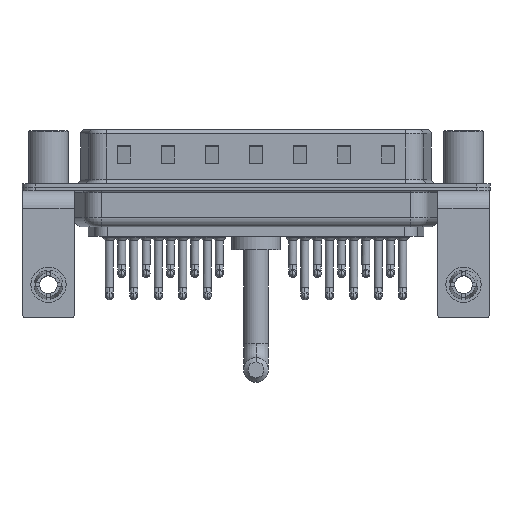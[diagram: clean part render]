
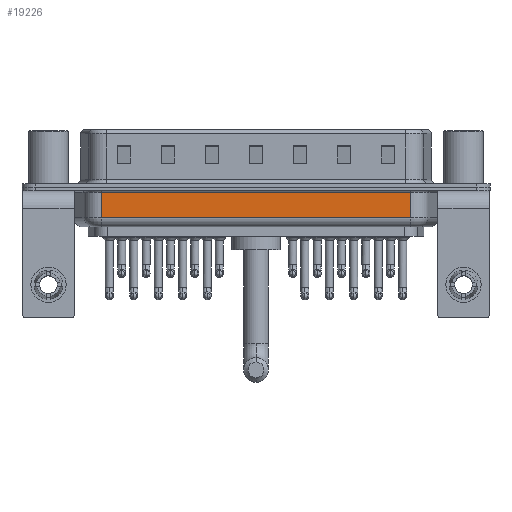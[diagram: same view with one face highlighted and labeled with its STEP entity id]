
A CAD part, front view. The second image highlights one B-rep face of the part: STEP entity #19226.
In plain terms, the highlighted planar face has unit normal (0, -1, 0).
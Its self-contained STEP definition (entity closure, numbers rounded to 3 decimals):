
#862 = VECTOR ( 'NONE', #10482, 1000. ) ;
#1079 = CARTESIAN_POINT ( 'NONE',  ( 6.006, -5.35, -4.5 ) ) ;
#1220 = LINE ( 'NONE', #22190, #28659 ) ;
#1743 = ORIENTED_EDGE ( 'NONE', *, *, #13119, .T. ) ;
#1830 = EDGE_CURVE ( 'NONE', #10763, #19965, #20393, .T. ) ;
#1931 = VECTOR ( 'NONE', #3828, 1000. ) ;
#3828 = DIRECTION ( 'NONE',  ( -1., 0., 0. ) ) ;
#9025 = DIRECTION ( 'NONE',  ( 1., 0., 0. ) ) ;
#9697 = CARTESIAN_POINT ( 'NONE',  ( 6.006, -5.35, -0.65 ) ) ;
#10061 = PLANE ( 'NONE',  #13688 ) ;
#10482 = DIRECTION ( 'NONE',  ( 0., 0., 1. ) ) ;
#10655 = DIRECTION ( 'NONE',  ( 0., 0., 1. ) ) ;
#10763 = VERTEX_POINT ( 'NONE', #20179 ) ;
#12751 = CARTESIAN_POINT ( 'NONE',  ( 41.044, -5.35, -4.5 ) ) ;
#13119 = EDGE_CURVE ( 'NONE', #27714, #25091, #13123, .T. ) ;
#13123 = LINE ( 'NONE', #29829, #19807 ) ;
#13688 = AXIS2_PLACEMENT_3D ( 'NONE', #1079, #19465, #10655 ) ;
#15354 = FACE_OUTER_BOUND ( 'NONE', #25283, .T. ) ;
#17093 = CARTESIAN_POINT ( 'NONE',  ( 41.044, -5.35, -3.5 ) ) ;
#17885 = EDGE_CURVE ( 'NONE', #27714, #19965, #1220, .T. ) ;
#18559 = CARTESIAN_POINT ( 'NONE',  ( 6.006, -5.35, -3.5 ) ) ;
#19226 = ADVANCED_FACE ( 'NONE', ( #15354 ), #10061, .F. ) ;
#19465 = DIRECTION ( 'NONE',  ( 0., 1., 0. ) ) ;
#19807 = VECTOR ( 'NONE', #9025, 1000. ) ;
#19965 = VERTEX_POINT ( 'NONE', #9697 ) ;
#20179 = CARTESIAN_POINT ( 'NONE',  ( 41.044, -5.35, -0.65 ) ) ;
#20194 = ORIENTED_EDGE ( 'NONE', *, *, #17885, .F. ) ;
#20393 = LINE ( 'NONE', #29654, #1931 ) ;
#21603 = DIRECTION ( 'NONE',  ( 0., 0., 1. ) ) ;
#22190 = CARTESIAN_POINT ( 'NONE',  ( 6.006, -5.35, -4.5 ) ) ;
#25091 = VERTEX_POINT ( 'NONE', #17093 ) ;
#25283 = EDGE_LOOP ( 'NONE', ( #20194, #1743, #28740, #29439 ) ) ;
#26567 = LINE ( 'NONE', #12751, #862 ) ;
#27714 = VERTEX_POINT ( 'NONE', #18559 ) ;
#28659 = VECTOR ( 'NONE', #21603, 1000. ) ;
#28740 = ORIENTED_EDGE ( 'NONE', *, *, #29735, .T. ) ;
#29439 = ORIENTED_EDGE ( 'NONE', *, *, #1830, .T. ) ;
#29654 = CARTESIAN_POINT ( 'NONE',  ( 6.006, -5.35, -0.65 ) ) ;
#29735 = EDGE_CURVE ( 'NONE', #25091, #10763, #26567, .T. ) ;
#29829 = CARTESIAN_POINT ( 'NONE',  ( 6.006, -5.35, -3.5 ) ) ;
